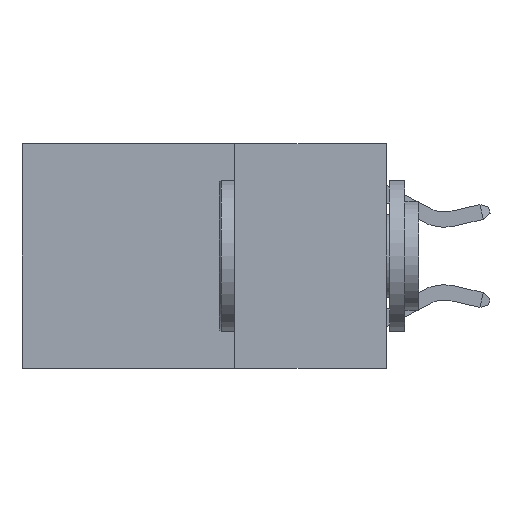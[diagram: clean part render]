
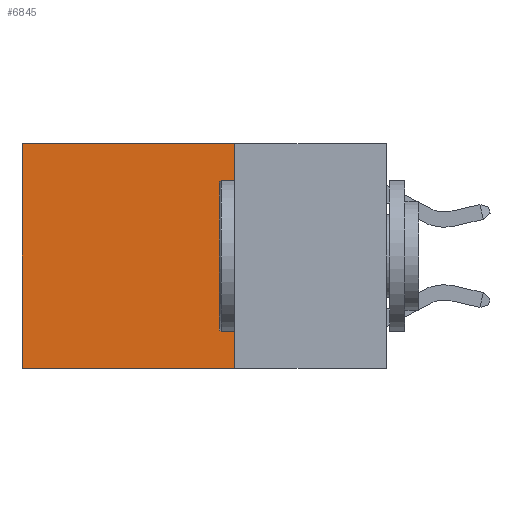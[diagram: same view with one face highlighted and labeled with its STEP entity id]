
A CAD part, left-side view. The second image highlights one B-rep face of the part: STEP entity #6845.
In plain terms, the highlighted planar face has unit normal (-1, 0, 0).
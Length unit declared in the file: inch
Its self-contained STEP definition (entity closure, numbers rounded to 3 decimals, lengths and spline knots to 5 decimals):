
#704 = CARTESIAN_POINT ( 'NONE',  ( 0.2625, 0.25, 0. ) ) ;
#1014 = LINE ( 'NONE', #6051, #2350 ) ;
#1050 = CARTESIAN_POINT ( 'NONE',  ( 0.2625, 0.6, 0. ) ) ;
#1151 = LINE ( 'NONE', #16655, #10996 ) ;
#2060 = ORIENTED_EDGE ( 'NONE', *, *, #14318, .T. ) ;
#2350 = VECTOR ( 'NONE', #11581, 39.37008 ) ;
#2466 = LINE ( 'NONE', #704, #8305 ) ;
#2762 = EDGE_LOOP ( 'NONE', ( #5660, #6693, #7560, #2060 ) ) ;
#3334 = VERTEX_POINT ( 'NONE', #7926 ) ;
#3773 = DIRECTION ( 'NONE',  ( 0., 1., 0. ) ) ;
#3871 = CARTESIAN_POINT ( 'NONE',  ( 0.2625, 0.6, -0.37 ) ) ;
#4611 = FACE_OUTER_BOUND ( 'NONE', #2762, .T. ) ;
#5660 = ORIENTED_EDGE ( 'NONE', *, *, #15325, .T. ) ;
#6051 = CARTESIAN_POINT ( 'NONE',  ( 0.2625, 0.25, -0.37 ) ) ;
#6590 = DIRECTION ( 'NONE',  ( 0., 0., -1. ) ) ;
#6693 = ORIENTED_EDGE ( 'NONE', *, *, #17706, .F. ) ;
#6714 = CARTESIAN_POINT ( 'NONE',  ( 0.2625, 0.25, 0. ) ) ;
#6845 = ADVANCED_FACE ( 'NONE', ( #4611 ), #17949, .F. ) ;
#6912 = CARTESIAN_POINT ( 'NONE',  ( 0.2625, 0.25, 0. ) ) ;
#7560 = ORIENTED_EDGE ( 'NONE', *, *, #14712, .F. ) ;
#7926 = CARTESIAN_POINT ( 'NONE',  ( 0.2625, 0.25, -0.37 ) ) ;
#8091 = DIRECTION ( 'NONE',  ( 0., 0., -1. ) ) ;
#8305 = VECTOR ( 'NONE', #8091, 39.37008 ) ;
#8588 = AXIS2_PLACEMENT_3D ( 'NONE', #6912, #13662, #6590 ) ;
#10996 = VECTOR ( 'NONE', #3773, 39.37008 ) ;
#11173 = LINE ( 'NONE', #1050, #12487 ) ;
#11581 = DIRECTION ( 'NONE',  ( 0., 1., 0. ) ) ;
#12487 = VECTOR ( 'NONE', #16614, 39.37008 ) ;
#13447 = VERTEX_POINT ( 'NONE', #14007 ) ;
#13662 = DIRECTION ( 'NONE',  ( 1., 0., 0. ) ) ;
#14007 = CARTESIAN_POINT ( 'NONE',  ( 0.2625, 0.6, 0. ) ) ;
#14318 = EDGE_CURVE ( 'NONE', #17883, #13447, #1151, .T. ) ;
#14712 = EDGE_CURVE ( 'NONE', #17883, #3334, #2466, .T. ) ;
#15325 = EDGE_CURVE ( 'NONE', #13447, #15717, #11173, .T. ) ;
#15717 = VERTEX_POINT ( 'NONE', #3871 ) ;
#16614 = DIRECTION ( 'NONE',  ( 0., 0., -1. ) ) ;
#16655 = CARTESIAN_POINT ( 'NONE',  ( 0.2625, 0.25, 0. ) ) ;
#17706 = EDGE_CURVE ( 'NONE', #3334, #15717, #1014, .T. ) ;
#17883 = VERTEX_POINT ( 'NONE', #6714 ) ;
#17949 = PLANE ( 'NONE',  #8588 ) ;
